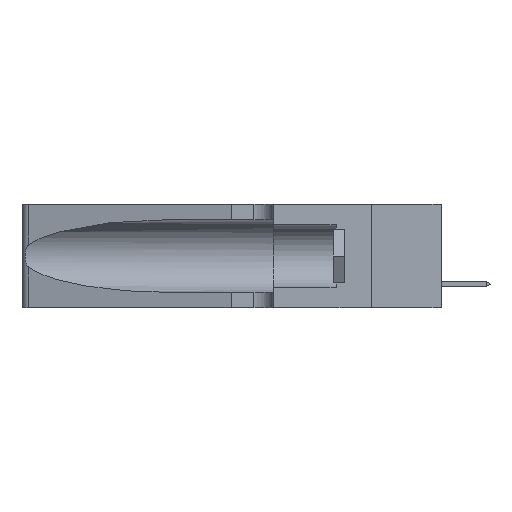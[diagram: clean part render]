
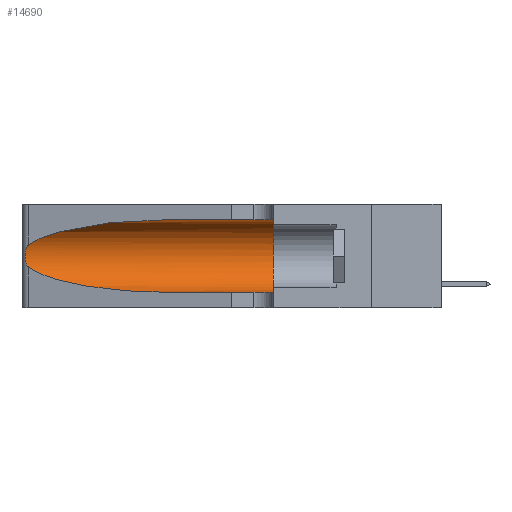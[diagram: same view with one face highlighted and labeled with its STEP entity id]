
A CAD part, left-side view. The second image highlights one B-rep face of the part: STEP entity #14690.
In plain terms, the highlighted cylindrical face has radius 3.308 mm (diameter 6.617 mm), a partial arc.
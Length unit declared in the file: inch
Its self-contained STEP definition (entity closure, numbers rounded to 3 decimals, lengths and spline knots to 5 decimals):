
#436 = DIRECTION ( 'NONE',  ( 0., 1., 0. ) ) ;
#674 = DIRECTION ( 'NONE',  ( 0., 0., 1. ) ) ;
#1418 = CARTESIAN_POINT ( 'NONE',  ( 0.25787, 1.23484, 0.2124 ) ) ;
#1500 = CARTESIAN_POINT ( 'NONE',  ( 0.25854, 1.2359, 0.20912 ) ) ;
#1734 = CARTESIAN_POINT ( 'NONE',  ( 0.1305, 0.35, 0.05475 ) ) ;
#2027 = VERTEX_POINT ( 'NONE', #18805 ) ;
#2125 = VERTEX_POINT ( 'NONE', #14809 ) ;
#3135 = CARTESIAN_POINT ( 'NONE',  ( 0.25555, 1.22993, 0.14849 ) ) ;
#3148 = CARTESIAN_POINT ( 'NONE',  ( 0.1305, 1.61858, 0.185 ) ) ;
#3285 = CARTESIAN_POINT ( 'NONE',  ( 0.26018, 1.23835, 0.19895 ) ) ;
#4387 = CARTESIAN_POINT ( 'NONE',  ( 0.2373, 1.15595, 0.08982 ) ) ;
#5369 = DIRECTION ( 'NONE',  ( 0., -1., 0. ) ) ;
#5647 = B_SPLINE_CURVE_WITH_KNOTS ( 'NONE', 3,
 ( #15835, #15751, #19789, #1418, #1500, #3285, #16075, #16240, #23456, #8739, #8972, #7134, #3135, #17931 ),
 .UNSPECIFIED., .F., .F.,
 ( 4, 2, 2, 2, 2, 2, 4 ),
 ( 0., 0.00027, 0.00053, 0.00107, 0.0016, 0.00187, 0.00214 ),
 .UNSPECIFIED. ) ;
#6018 = CARTESIAN_POINT ( 'NONE',  ( 0.2373, 1.15595, 0.28018 ) ) ;
#6140 = DIRECTION ( 'NONE',  ( 0., -1., 0. ) ) ;
#6411 =( BOUNDED_CURVE ( )  B_SPLINE_CURVE ( 3, ( #8068, #18346, #6018, #20849 ),
 .UNSPECIFIED., .F., .T. ) 
 B_SPLINE_CURVE_WITH_KNOTS ( ( 4, 4 ),
 ( 1.5708, 2.84003 ),
 .UNSPECIFIED. ) 
 CURVE ( )  GEOMETRIC_REPRESENTATION_ITEM ( )  RATIONAL_B_SPLINE_CURVE ( ( 1., 0.87, 0.87, 1. ) ) 
 REPRESENTATION_ITEM ( '' )  );
#6709 = VERTEX_POINT ( 'NONE', #1734 ) ;
#6966 = VECTOR ( 'NONE', #14285, 39.37008 ) ;
#7134 = CARTESIAN_POINT ( 'NONE',  ( 0.25639, 1.23186, 0.15144 ) ) ;
#7999 = AXIS2_PLACEMENT_3D ( 'NONE', #15126, #436, #674 ) ;
#8037 = CARTESIAN_POINT ( 'NONE',  ( 0.25487, 1.22718, 0.14631 ) ) ;
#8068 = CARTESIAN_POINT ( 'NONE',  ( 0.1305, 0.72297, 0.31525 ) ) ;
#8155 = FACE_OUTER_BOUND ( 'NONE', #19737, .T. ) ;
#8256 = ORIENTED_EDGE ( 'NONE', *, *, #15092, .T. ) ;
#8459 = EDGE_CURVE ( 'NONE', #19647, #6709, #9784, .T. ) ;
#8739 = CARTESIAN_POINT ( 'NONE',  ( 0.25856, 1.23593, 0.16098 ) ) ;
#8972 = CARTESIAN_POINT ( 'NONE',  ( 0.25789, 1.23486, 0.15765 ) ) ;
#8991 = CYLINDRICAL_SURFACE ( 'NONE', #10978, 0.13025 ) ;
#9292 = VERTEX_POINT ( 'NONE', #16798 ) ;
#9784 = LINE ( 'NONE', #20897, #15841 ) ;
#9997 = ORIENTED_EDGE ( 'NONE', *, *, #20910, .F. ) ;
#10978 = AXIS2_PLACEMENT_3D ( 'NONE', #3148, #5369, #23903 ) ;
#11891 = EDGE_CURVE ( 'NONE', #2027, #19647, #23296, .T. ) ;
#12278 = CARTESIAN_POINT ( 'NONE',  ( 0.1305, 0.35, 0.31525 ) ) ;
#12469 = CARTESIAN_POINT ( 'NONE',  ( 0.1305, 1.61858, 0.31525 ) ) ;
#12948 = ORIENTED_EDGE ( 'NONE', *, *, #21791, .T. ) ;
#13133 = CIRCLE ( 'NONE', #7999, 0.13025 ) ;
#13215 = CARTESIAN_POINT ( 'NONE',  ( 0.1305, 0.72297, 0.05475 ) ) ;
#13459 = ORIENTED_EDGE ( 'NONE', *, *, #8459, .T. ) ;
#14285 = DIRECTION ( 'NONE',  ( 0., -1., 0. ) ) ;
#14690 = ADVANCED_FACE ( 'NONE', ( #8155 ), #8991, .F. ) ;
#14809 = CARTESIAN_POINT ( 'NONE',  ( 0.1305, 0.72297, 0.31525 ) ) ;
#15067 = EDGE_CURVE ( 'NONE', #2125, #23386, #15315, .T. ) ;
#15092 = EDGE_CURVE ( 'NONE', #2125, #9292, #6411, .T. ) ;
#15126 = CARTESIAN_POINT ( 'NONE',  ( 0.1305, 0.35, 0.185 ) ) ;
#15315 = LINE ( 'NONE', #12469, #6966 ) ;
#15685 = ORIENTED_EDGE ( 'NONE', *, *, #15067, .F. ) ;
#15751 = CARTESIAN_POINT ( 'NONE',  ( 0.25555, 1.22994, 0.2215 ) ) ;
#15778 = CARTESIAN_POINT ( 'NONE',  ( 0.1305, 0.72297, 0.05475 ) ) ;
#15835 = CARTESIAN_POINT ( 'NONE',  ( 0.25487, 1.22718, 0.22369 ) ) ;
#15841 = VECTOR ( 'NONE', #6140, 39.37008 ) ;
#16075 = CARTESIAN_POINT ( 'NONE',  ( 0.26075, 1.23896, 0.19203 ) ) ;
#16240 = CARTESIAN_POINT ( 'NONE',  ( 0.26075, 1.23896, 0.178 ) ) ;
#16798 = CARTESIAN_POINT ( 'NONE',  ( 0.25487, 1.22718, 0.22369 ) ) ;
#17313 = CARTESIAN_POINT ( 'NONE',  ( 0.18966, 0.96281, 0.05475 ) ) ;
#17931 = CARTESIAN_POINT ( 'NONE',  ( 0.25487, 1.22718, 0.14631 ) ) ;
#18346 = CARTESIAN_POINT ( 'NONE',  ( 0.18966, 0.96281, 0.31525 ) ) ;
#18805 = CARTESIAN_POINT ( 'NONE',  ( 0.25487, 1.22718, 0.14631 ) ) ;
#18816 = ORIENTED_EDGE ( 'NONE', *, *, #11891, .T. ) ;
#19647 = VERTEX_POINT ( 'NONE', #15778 ) ;
#19737 = EDGE_LOOP ( 'NONE', ( #8256, #12948, #18816, #13459, #9997, #15685 ) ) ;
#19789 = CARTESIAN_POINT ( 'NONE',  ( 0.25639, 1.23184, 0.21858 ) ) ;
#20849 = CARTESIAN_POINT ( 'NONE',  ( 0.25487, 1.22718, 0.22369 ) ) ;
#20897 = CARTESIAN_POINT ( 'NONE',  ( 0.1305, 1.61858, 0.05475 ) ) ;
#20910 = EDGE_CURVE ( 'NONE', #23386, #6709, #13133, .T. ) ;
#21791 = EDGE_CURVE ( 'NONE', #9292, #2027, #5647, .T. ) ;
#23296 =( BOUNDED_CURVE ( )  B_SPLINE_CURVE ( 3, ( #8037, #4387, #17313, #13215 ),
 .UNSPECIFIED., .F., .T. ) 
 B_SPLINE_CURVE_WITH_KNOTS ( ( 4, 4 ),
 ( 3.44316, 4.71239 ),
 .UNSPECIFIED. ) 
 CURVE ( )  GEOMETRIC_REPRESENTATION_ITEM ( )  RATIONAL_B_SPLINE_CURVE ( ( 1., 0.87, 0.87, 1. ) ) 
 REPRESENTATION_ITEM ( '' )  );
#23386 = VERTEX_POINT ( 'NONE', #12278 ) ;
#23456 = CARTESIAN_POINT ( 'NONE',  ( 0.26017, 1.23833, 0.17102 ) ) ;
#23903 = DIRECTION ( 'NONE',  ( 0., 0., -1. ) ) ;
